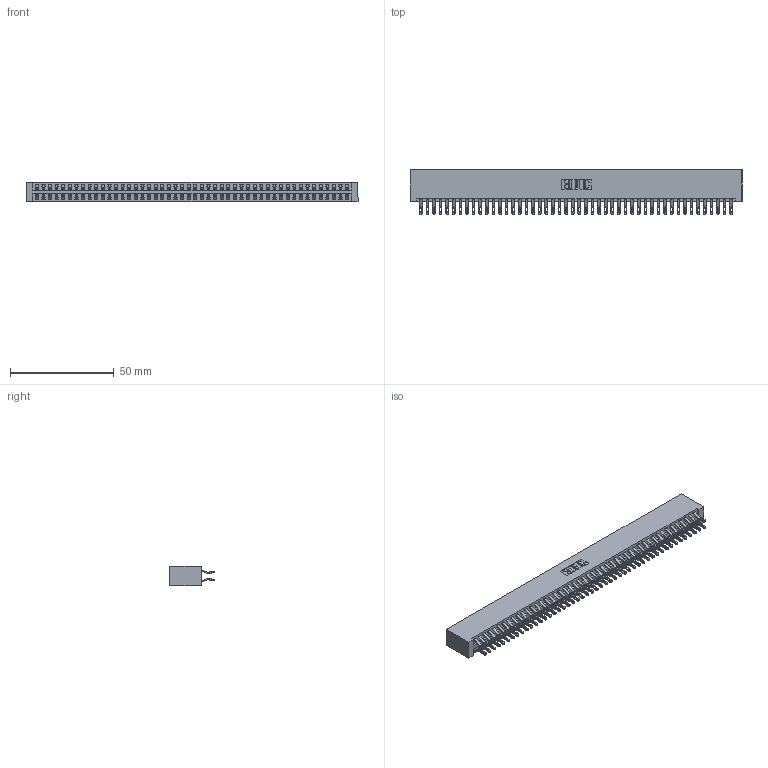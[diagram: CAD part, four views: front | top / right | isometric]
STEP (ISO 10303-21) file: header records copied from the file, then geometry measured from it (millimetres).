
FILE_DESCRIPTION (( 'STEP AP203' ), '1' );
FILE_NAME ('346-096-555-201.STEP', '2022-05-26T16:39:33', ( '' ), ( '' ), 'SwSTEP 2.0', 'SolidWorks 2020', '' );
FILE_SCHEMA (( 'CONFIG_CONTROL_DESIGN' ));
Length unit declared in the file: inch
Products named in the file (3): 345-292-001_555 Tail; 346 Part_No Mounting Lugs; 346-096-555-201
Assembly tree (97 placements, depth 2):
  346-096-555-201
    346 Part_No Mounting Lugs
    345-292-001_555 Tail  x96
Bounding box: 159.64 x 21.46 x 9.4 mm (x, y, z)
Volume: 16465.1 mm3; surface area: 23882.5 mm2
Topology: 97 solids, 97 shells, 5682 faces, 17873 edges, 11914 vertices
Faces by surface type: plane 3240, cylinder 2442
Entity records: 30567 total; most frequent: CARTESIAN_POINT 5062, ORIENTED_EDGE 4966, DIRECTION 4475, EDGE_CURVE 2483, LINE 2147, VECTOR 2147, VERTEX_POINT 1654, AXIS2_PLACEMENT_3D 1164
